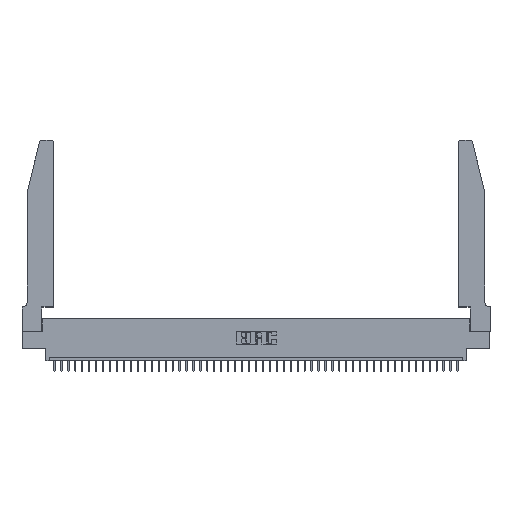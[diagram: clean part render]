
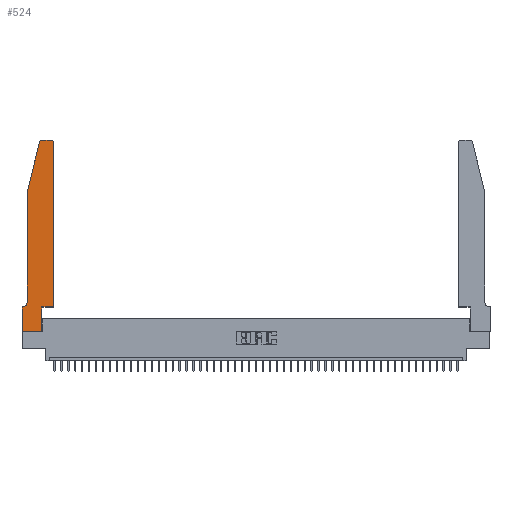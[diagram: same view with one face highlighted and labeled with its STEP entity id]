
A CAD part, top view. The second image highlights one B-rep face of the part: STEP entity #524.
In plain terms, the highlighted planar face has unit normal (0, 0, 1).
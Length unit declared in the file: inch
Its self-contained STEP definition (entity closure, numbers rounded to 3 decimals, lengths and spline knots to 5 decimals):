
#13 = CARTESIAN_POINT ( 'NONE',  ( 0.2605, 2.75, 0.37 ) ) ;
#524 = ADVANCED_FACE ( 'NONE', ( #22555 ), #20923, .T. ) ;
#738 = CARTESIAN_POINT ( 'NONE',  ( 0.0055, 0.42, 0.37 ) ) ;
#1248 = ORIENTED_EDGE ( 'NONE', *, *, #26004, .T. ) ;
#2052 = VECTOR ( 'NONE', #22075, 39.37008 ) ;
#3125 = CARTESIAN_POINT ( 'NONE',  ( 0.4505, 0.35, 0.37 ) ) ;
#3189 = EDGE_CURVE ( 'NONE', #12527, #28417, #15558, .T. ) ;
#3206 = CARTESIAN_POINT ( 'NONE',  ( 0., 0., 0.37 ) ) ;
#4084 = DIRECTION ( 'NONE',  ( 0., 0., -1. ) ) ;
#4624 = CARTESIAN_POINT ( 'NONE',  ( 0.2865, 0.35, 0.37 ) ) ;
#5768 = CARTESIAN_POINT ( 'NONE',  ( 0.0755, 2., 0.37 ) ) ;
#5921 = CARTESIAN_POINT ( 'NONE',  ( 0.4205, 2.75, 0.37 ) ) ;
#6061 = VECTOR ( 'NONE', #45529, 39.37008 ) ;
#6170 = ORIENTED_EDGE ( 'NONE', *, *, #34635, .T. ) ;
#6193 = EDGE_LOOP ( 'NONE', ( #27247, #24777, #15038, #44100, #29957, #1248, #28784, #35782, #46691, #6697, #6170, #42001 ) ) ;
#6658 = DIRECTION ( 'NONE',  ( 0., 1., 0. ) ) ;
#6697 = ORIENTED_EDGE ( 'NONE', *, *, #13783, .T. ) ;
#7494 = VECTOR ( 'NONE', #46008, 39.37008 ) ;
#8392 = EDGE_CURVE ( 'NONE', #45545, #27807, #34667, .T. ) ;
#8612 = CARTESIAN_POINT ( 'NONE',  ( 0.284, 2.72, 0.37 ) ) ;
#9242 = AXIS2_PLACEMENT_3D ( 'NONE', #14888, #41251, #41104 ) ;
#10132 = CARTESIAN_POINT ( 'NONE',  ( 0., 0.35, 0.37 ) ) ;
#10212 = CARTESIAN_POINT ( 'NONE',  ( 0.0755, 0.42, 0.37 ) ) ;
#10459 = EDGE_CURVE ( 'NONE', #37585, #18397, #21454, .T. ) ;
#10481 = DIRECTION ( 'NONE',  ( 0., 0., 1. ) ) ;
#11067 = CARTESIAN_POINT ( 'NONE',  ( 0.0755, 2., 0.37 ) ) ;
#11164 = CARTESIAN_POINT ( 'NONE',  ( 0.0755, 0.35, 0.37 ) ) ;
#12527 = VERTEX_POINT ( 'NONE', #5921 ) ;
#13164 = VECTOR ( 'NONE', #24821, 39.37008 ) ;
#13783 = EDGE_CURVE ( 'NONE', #18397, #38161, #23961, .T. ) ;
#13805 = VERTEX_POINT ( 'NONE', #10132 ) ;
#13910 = EDGE_CURVE ( 'NONE', #33235, #37585, #36467, .T. ) ;
#14095 = CARTESIAN_POINT ( 'NONE',  ( 0.2865, 0.35, 0.37 ) ) ;
#14888 = CARTESIAN_POINT ( 'NONE',  ( 0.4205, 2.72, 0.37 ) ) ;
#15038 = ORIENTED_EDGE ( 'NONE', *, *, #8392, .T. ) ;
#15237 = VERTEX_POINT ( 'NONE', #45130 ) ;
#15270 = AXIS2_PLACEMENT_3D ( 'NONE', #32220, #10481, #25223 ) ;
#15558 = LINE ( 'NONE', #13, #37152 ) ;
#15668 = CARTESIAN_POINT ( 'NONE',  ( 0.4505, 2.72, 0.37 ) ) ;
#17042 = CARTESIAN_POINT ( 'NONE',  ( 0.4505, 0.35, 0.37 ) ) ;
#17257 = CARTESIAN_POINT ( 'NONE',  ( 0.2865, 0., 0.37 ) ) ;
#18148 = CARTESIAN_POINT ( 'NONE',  ( 0.25487, 2.72718, 0.37 ) ) ;
#18397 = VERTEX_POINT ( 'NONE', #4624 ) ;
#20114 = CARTESIAN_POINT ( 'NONE',  ( 0., 0., 0.37 ) ) ;
#20923 = PLANE ( 'NONE',  #15270 ) ;
#20974 = DIRECTION ( 'NONE',  ( 0., -1., 0. ) ) ;
#21454 = LINE ( 'NONE', #14095, #27175 ) ;
#22075 = DIRECTION ( 'NONE',  ( -1., 0., 0. ) ) ;
#22413 = AXIS2_PLACEMENT_3D ( 'NONE', #8612, #26689, #22704 ) ;
#22485 = LINE ( 'NONE', #11164, #2052 ) ;
#22555 = FACE_OUTER_BOUND ( 'NONE', #6193, .T. ) ;
#22704 = DIRECTION ( 'NONE',  ( 1., 0., 0. ) ) ;
#23298 = EDGE_CURVE ( 'NONE', #13805, #33235, #37314, .T. ) ;
#23872 = VECTOR ( 'NONE', #29932, 39.37008 ) ;
#23961 = LINE ( 'NONE', #31250, #7494 ) ;
#24777 = ORIENTED_EDGE ( 'NONE', *, *, #29704, .T. ) ;
#24821 = DIRECTION ( 'NONE',  ( 1., 0., 0. ) ) ;
#24974 = EDGE_CURVE ( 'NONE', #35952, #12527, #38348, .T. ) ;
#25223 = DIRECTION ( 'NONE',  ( 1., 0., 0. ) ) ;
#25435 = CARTESIAN_POINT ( 'NONE',  ( 0.284, 2.75, 0.37 ) ) ;
#26004 = EDGE_CURVE ( 'NONE', #15237, #13805, #22485, .T. ) ;
#26689 = DIRECTION ( 'NONE',  ( 0., 0., 1. ) ) ;
#27175 = VECTOR ( 'NONE', #6658, 39.37008 ) ;
#27247 = ORIENTED_EDGE ( 'NONE', *, *, #3189, .T. ) ;
#27807 = VERTEX_POINT ( 'NONE', #11067 ) ;
#28417 = VERTEX_POINT ( 'NONE', #25435 ) ;
#28784 = ORIENTED_EDGE ( 'NONE', *, *, #23298, .T. ) ;
#29145 = EDGE_CURVE ( 'NONE', #39523, #15237, #29716, .T. ) ;
#29315 = CARTESIAN_POINT ( 'NONE',  ( 0.0755, 2., 0.37 ) ) ;
#29493 = DIRECTION ( 'NONE',  ( -1., 0., 0. ) ) ;
#29704 = EDGE_CURVE ( 'NONE', #28417, #45545, #31926, .T. ) ;
#29716 = CIRCLE ( 'NONE', #30004, 0.07 ) ;
#29932 = DIRECTION ( 'NONE',  ( -0.239, -0.971, 0. ) ) ;
#29957 = ORIENTED_EDGE ( 'NONE', *, *, #29145, .T. ) ;
#30004 = AXIS2_PLACEMENT_3D ( 'NONE', #738, #4084, #29493 ) ;
#31250 = CARTESIAN_POINT ( 'NONE',  ( 0.4505, 0.35, 0.37 ) ) ;
#31926 = CIRCLE ( 'NONE', #22413, 0.03 ) ;
#32220 = CARTESIAN_POINT ( 'NONE',  ( 0., 0.35, 0.37 ) ) ;
#33235 = VERTEX_POINT ( 'NONE', #38061 ) ;
#33874 = VECTOR ( 'NONE', #46174, 39.37008 ) ;
#34635 = EDGE_CURVE ( 'NONE', #38161, #35952, #37874, .T. ) ;
#34667 = LINE ( 'NONE', #29315, #23872 ) ;
#35782 = ORIENTED_EDGE ( 'NONE', *, *, #13910, .T. ) ;
#35952 = VERTEX_POINT ( 'NONE', #15668 ) ;
#36467 = LINE ( 'NONE', #3206, #13164 ) ;
#36859 = DIRECTION ( 'NONE',  ( -1., 0., 0. ) ) ;
#37152 = VECTOR ( 'NONE', #36859, 39.37008 ) ;
#37314 = LINE ( 'NONE', #20114, #6061 ) ;
#37585 = VERTEX_POINT ( 'NONE', #17257 ) ;
#37874 = LINE ( 'NONE', #3125, #33874 ) ;
#38061 = CARTESIAN_POINT ( 'NONE',  ( 0., 0., 0.37 ) ) ;
#38161 = VERTEX_POINT ( 'NONE', #17042 ) ;
#38222 = LINE ( 'NONE', #5768, #41628 ) ;
#38348 = CIRCLE ( 'NONE', #9242, 0.03 ) ;
#39523 = VERTEX_POINT ( 'NONE', #10212 ) ;
#41104 = DIRECTION ( 'NONE',  ( 1., 0., 0. ) ) ;
#41251 = DIRECTION ( 'NONE',  ( 0., 0., 1. ) ) ;
#41271 = EDGE_CURVE ( 'NONE', #27807, #39523, #38222, .T. ) ;
#41628 = VECTOR ( 'NONE', #20974, 39.37008 ) ;
#42001 = ORIENTED_EDGE ( 'NONE', *, *, #24974, .T. ) ;
#44100 = ORIENTED_EDGE ( 'NONE', *, *, #41271, .T. ) ;
#45130 = CARTESIAN_POINT ( 'NONE',  ( 0.0055, 0.35, 0.37 ) ) ;
#45529 = DIRECTION ( 'NONE',  ( 0., -1., 0. ) ) ;
#45545 = VERTEX_POINT ( 'NONE', #18148 ) ;
#46008 = DIRECTION ( 'NONE',  ( 1., 0., 0. ) ) ;
#46174 = DIRECTION ( 'NONE',  ( 0., 1., 0. ) ) ;
#46691 = ORIENTED_EDGE ( 'NONE', *, *, #10459, .T. ) ;
